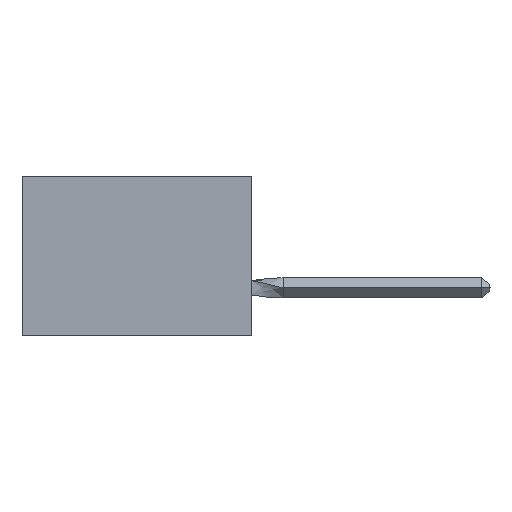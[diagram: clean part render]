
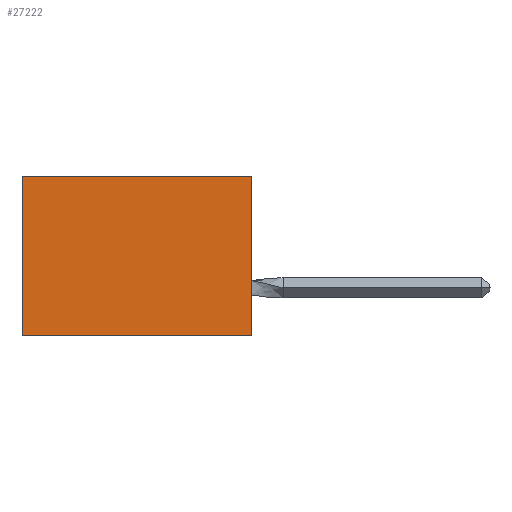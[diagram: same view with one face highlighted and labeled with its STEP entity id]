
A CAD part, left-side view. The second image highlights one B-rep face of the part: STEP entity #27222.
In plain terms, the highlighted planar face has unit normal (-1, 0, 0).
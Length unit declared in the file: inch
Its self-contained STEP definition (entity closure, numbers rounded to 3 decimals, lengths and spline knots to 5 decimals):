
#61 = VERTEX_POINT ( 'NONE', #22027 ) ;
#272 = CARTESIAN_POINT ( 'NONE',  ( 0.305, 0.72, -0.5 ) ) ;
#1795 = DIRECTION ( 'NONE',  ( 0., 0., -1. ) ) ;
#1990 = EDGE_LOOP ( 'NONE', ( #10714, #3039, #7020, #14158 ) ) ;
#3016 = LINE ( 'NONE', #20692, #16544 ) ;
#3039 = ORIENTED_EDGE ( 'NONE', *, *, #14664, .F. ) ;
#3853 = LINE ( 'NONE', #26041, #8042 ) ;
#4105 = DIRECTION ( 'NONE',  ( 1., 0., 0. ) ) ;
#4637 = VERTEX_POINT ( 'NONE', #13178 ) ;
#6012 = VERTEX_POINT ( 'NONE', #272 ) ;
#7020 = ORIENTED_EDGE ( 'NONE', *, *, #23663, .F. ) ;
#7102 = CARTESIAN_POINT ( 'NONE',  ( 0.305, 0., 0. ) ) ;
#7371 = CARTESIAN_POINT ( 'NONE',  ( 0.305, 0.72, -0.5 ) ) ;
#8042 = VECTOR ( 'NONE', #10622, 39.37008 ) ;
#10622 = DIRECTION ( 'NONE',  ( 0., 1., 0. ) ) ;
#10714 = ORIENTED_EDGE ( 'NONE', *, *, #20984, .T. ) ;
#10794 = CARTESIAN_POINT ( 'NONE',  ( 0.305, 0., -0.5 ) ) ;
#11889 = DIRECTION ( 'NONE',  ( 0., 1., 0. ) ) ;
#13178 = CARTESIAN_POINT ( 'NONE',  ( 0.305, 0., -0.5 ) ) ;
#14158 = ORIENTED_EDGE ( 'NONE', *, *, #17921, .T. ) ;
#14259 = VECTOR ( 'NONE', #18957, 39.37008 ) ;
#14664 = EDGE_CURVE ( 'NONE', #4637, #6012, #3853, .T. ) ;
#14790 = FACE_OUTER_BOUND ( 'NONE', #1990, .T. ) ;
#16376 = DIRECTION ( 'NONE',  ( 0., 0., -1. ) ) ;
#16544 = VECTOR ( 'NONE', #11889, 39.37008 ) ;
#17921 = EDGE_CURVE ( 'NONE', #20348, #61, #3016, .T. ) ;
#18655 = AXIS2_PLACEMENT_3D ( 'NONE', #10794, #4105, #1795 ) ;
#18957 = DIRECTION ( 'NONE',  ( 0., 0., -1. ) ) ;
#20348 = VERTEX_POINT ( 'NONE', #7102 ) ;
#20692 = CARTESIAN_POINT ( 'NONE',  ( 0.305, 0., 0. ) ) ;
#20984 = EDGE_CURVE ( 'NONE', #61, #6012, #28175, .T. ) ;
#21519 = LINE ( 'NONE', #23398, #14259 ) ;
#21642 = VECTOR ( 'NONE', #16376, 39.37008 ) ;
#22027 = CARTESIAN_POINT ( 'NONE',  ( 0.305, 0.72, 0. ) ) ;
#23398 = CARTESIAN_POINT ( 'NONE',  ( 0.305, 0., -0.5 ) ) ;
#23663 = EDGE_CURVE ( 'NONE', #20348, #4637, #21519, .T. ) ;
#26041 = CARTESIAN_POINT ( 'NONE',  ( 0.305, 0., -0.5 ) ) ;
#27222 = ADVANCED_FACE ( 'NONE', ( #14790 ), #28540, .F. ) ;
#28175 = LINE ( 'NONE', #7371, #21642 ) ;
#28540 = PLANE ( 'NONE',  #18655 ) ;
